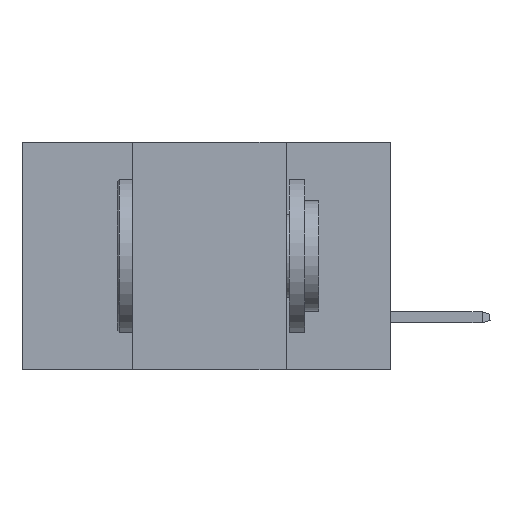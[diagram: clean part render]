
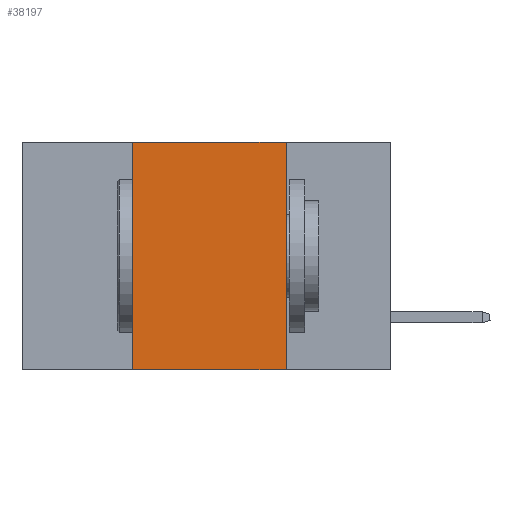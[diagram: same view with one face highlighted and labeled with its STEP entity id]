
A CAD part, left-side view. The second image highlights one B-rep face of the part: STEP entity #38197.
In plain terms, the highlighted planar face has unit normal (-1, 0, 0).
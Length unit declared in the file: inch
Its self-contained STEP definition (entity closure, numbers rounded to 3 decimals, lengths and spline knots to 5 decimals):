
#922 = VERTEX_POINT ( 'NONE', #31685 ) ;
#2729 = CARTESIAN_POINT ( 'NONE',  ( 0., 0.42, 0. ) ) ;
#4099 = EDGE_CURVE ( 'NONE', #6226, #922, #28957, .T. ) ;
#6226 = VERTEX_POINT ( 'NONE', #2729 ) ;
#6366 = CARTESIAN_POINT ( 'NONE',  ( 0., 0.6, 0. ) ) ;
#7261 = CARTESIAN_POINT ( 'NONE',  ( 0., 0.42, 0. ) ) ;
#7901 = EDGE_CURVE ( 'NONE', #922, #8819, #33178, .T. ) ;
#8819 = VERTEX_POINT ( 'NONE', #20743 ) ;
#9969 = EDGE_CURVE ( 'NONE', #29765, #6226, #29277, .T. ) ;
#10166 = CARTESIAN_POINT ( 'NONE',  ( 0., 0.42, -0.37 ) ) ;
#10274 = CARTESIAN_POINT ( 'NONE',  ( 0., 0.6, 0. ) ) ;
#10310 = DIRECTION ( 'NONE',  ( 0., -1., 0. ) ) ;
#12629 = PLANE ( 'NONE',  #33550 ) ;
#13299 = ORIENTED_EDGE ( 'NONE', *, *, #9969, .F. ) ;
#15022 = CARTESIAN_POINT ( 'NONE',  ( 0., 0.6, -0.37 ) ) ;
#15723 = ORIENTED_EDGE ( 'NONE', *, *, #4099, .F. ) ;
#15754 = DIRECTION ( 'NONE',  ( 1., 0., 0. ) ) ;
#16396 = CARTESIAN_POINT ( 'NONE',  ( 0., 0.17, 0. ) ) ;
#20743 = CARTESIAN_POINT ( 'NONE',  ( 0., 0.17, -0.37 ) ) ;
#22551 = DIRECTION ( 'NONE',  ( 0., 0., -1. ) ) ;
#23381 = ORIENTED_EDGE ( 'NONE', *, *, #7901, .F. ) ;
#24787 = EDGE_CURVE ( 'NONE', #29765, #8819, #30112, .T. ) ;
#26268 = FACE_OUTER_BOUND ( 'NONE', #28386, .T. ) ;
#28386 = EDGE_LOOP ( 'NONE', ( #23381, #15723, #13299, #37270 ) ) ;
#28957 = LINE ( 'NONE', #10274, #36095 ) ;
#29277 = LINE ( 'NONE', #7261, #36406 ) ;
#29765 = VERTEX_POINT ( 'NONE', #10166 ) ;
#30112 = LINE ( 'NONE', #15022, #37243 ) ;
#31685 = CARTESIAN_POINT ( 'NONE',  ( 0., 0.17, 0. ) ) ;
#31900 = DIRECTION ( 'NONE',  ( 0., 0., 1. ) ) ;
#32222 = VECTOR ( 'NONE', #22551, 39.37008 ) ;
#33178 = LINE ( 'NONE', #16396, #32222 ) ;
#33365 = DIRECTION ( 'NONE',  ( 0., -1., 0. ) ) ;
#33550 = AXIS2_PLACEMENT_3D ( 'NONE', #6366, #15754, #37146 ) ;
#36095 = VECTOR ( 'NONE', #10310, 39.37008 ) ;
#36406 = VECTOR ( 'NONE', #31900, 39.37008 ) ;
#37146 = DIRECTION ( 'NONE',  ( 0., 0., -1. ) ) ;
#37243 = VECTOR ( 'NONE', #33365, 39.37008 ) ;
#37270 = ORIENTED_EDGE ( 'NONE', *, *, #24787, .T. ) ;
#38197 = ADVANCED_FACE ( 'NONE', ( #26268 ), #12629, .F. ) ;
